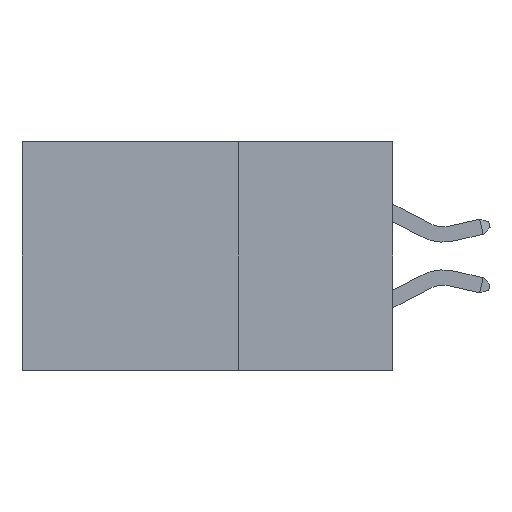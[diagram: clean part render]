
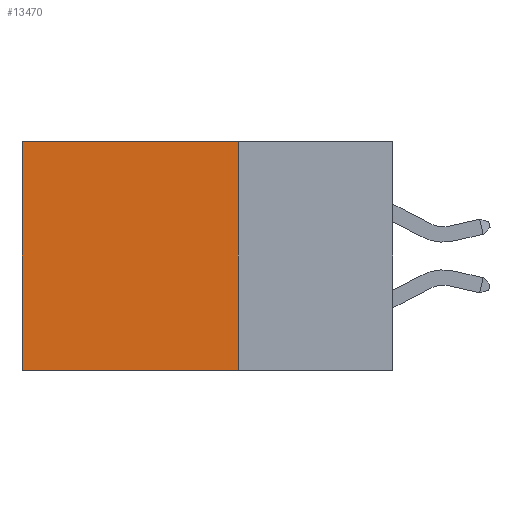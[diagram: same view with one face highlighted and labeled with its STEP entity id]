
A CAD part, left-side view. The second image highlights one B-rep face of the part: STEP entity #13470.
In plain terms, the highlighted planar face has unit normal (-1, 0, 0).
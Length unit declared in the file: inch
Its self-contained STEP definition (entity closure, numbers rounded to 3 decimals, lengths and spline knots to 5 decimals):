
#1354 = AXIS2_PLACEMENT_3D ( 'NONE', #4075, #13843, #23444 ) ;
#2212 = LINE ( 'NONE', #17244, #20484 ) ;
#2810 = LINE ( 'NONE', #16754, #23340 ) ;
#3268 = LINE ( 'NONE', #15594, #26530 ) ;
#3864 = ORIENTED_EDGE ( 'NONE', *, *, #30219, .T. ) ;
#4075 = CARTESIAN_POINT ( 'NONE',  ( 0.2875, 0.25, 0. ) ) ;
#5894 = VERTEX_POINT ( 'NONE', #30977 ) ;
#8992 = ORIENTED_EDGE ( 'NONE', *, *, #25703, .F. ) ;
#9517 = VERTEX_POINT ( 'NONE', #14140 ) ;
#9758 = DIRECTION ( 'NONE',  ( 0., 1., 0. ) ) ;
#10175 = CARTESIAN_POINT ( 'NONE',  ( 0.2875, 0.6, -0.37 ) ) ;
#10642 = DIRECTION ( 'NONE',  ( 0., 0., -1. ) ) ;
#12874 = DIRECTION ( 'NONE',  ( 0., 1., 0. ) ) ;
#13470 = ADVANCED_FACE ( 'NONE', ( #26173 ), #13680, .F. ) ;
#13680 = PLANE ( 'NONE',  #1354 ) ;
#13843 = DIRECTION ( 'NONE',  ( 1., 0., 0. ) ) ;
#13920 = CARTESIAN_POINT ( 'NONE',  ( 0.2875, 0.25, 0. ) ) ;
#14140 = CARTESIAN_POINT ( 'NONE',  ( 0.2875, 0.6, 0. ) ) ;
#15388 = VECTOR ( 'NONE', #12874, 39.37008 ) ;
#15594 = CARTESIAN_POINT ( 'NONE',  ( 0.2875, 0.25, 0. ) ) ;
#16754 = CARTESIAN_POINT ( 'NONE',  ( 0.2875, 0.6, 0. ) ) ;
#17244 = CARTESIAN_POINT ( 'NONE',  ( 0.2875, 0.25, -0.37 ) ) ;
#17664 = ORIENTED_EDGE ( 'NONE', *, *, #23369, .T. ) ;
#20237 = VERTEX_POINT ( 'NONE', #13920 ) ;
#20425 = ORIENTED_EDGE ( 'NONE', *, *, #29496, .F. ) ;
#20484 = VECTOR ( 'NONE', #9758, 39.37008 ) ;
#21192 = EDGE_LOOP ( 'NONE', ( #17664, #20425, #8992, #3864 ) ) ;
#22790 = CARTESIAN_POINT ( 'NONE',  ( 0.2875, 0.25, 0. ) ) ;
#23340 = VECTOR ( 'NONE', #26538, 39.37008 ) ;
#23369 = EDGE_CURVE ( 'NONE', #9517, #28237, #2810, .T. ) ;
#23444 = DIRECTION ( 'NONE',  ( 0., 0., -1. ) ) ;
#25703 = EDGE_CURVE ( 'NONE', #20237, #5894, #3268, .T. ) ;
#26173 = FACE_OUTER_BOUND ( 'NONE', #21192, .T. ) ;
#26530 = VECTOR ( 'NONE', #10642, 39.37008 ) ;
#26538 = DIRECTION ( 'NONE',  ( 0., 0., -1. ) ) ;
#27123 = LINE ( 'NONE', #22790, #15388 ) ;
#28237 = VERTEX_POINT ( 'NONE', #10175 ) ;
#29496 = EDGE_CURVE ( 'NONE', #5894, #28237, #2212, .T. ) ;
#30219 = EDGE_CURVE ( 'NONE', #20237, #9517, #27123, .T. ) ;
#30977 = CARTESIAN_POINT ( 'NONE',  ( 0.2875, 0.25, -0.37 ) ) ;
